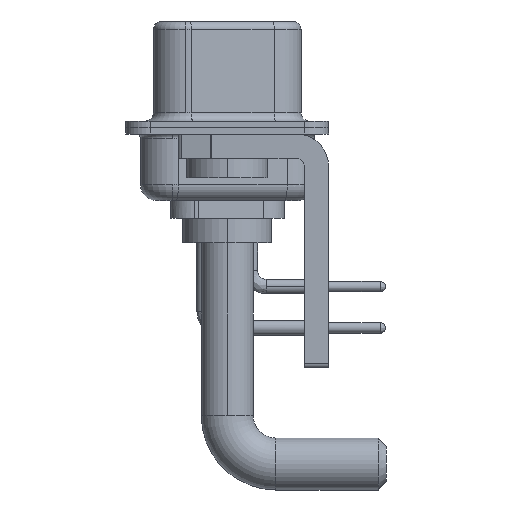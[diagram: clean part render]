
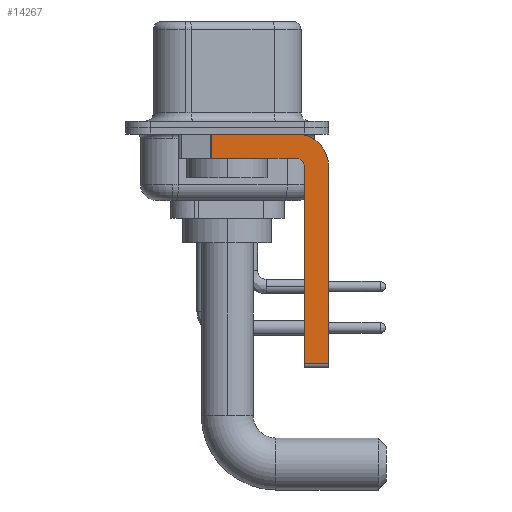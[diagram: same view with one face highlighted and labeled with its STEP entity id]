
A CAD part, left-side view. The second image highlights one B-rep face of the part: STEP entity #14267.
In plain terms, the highlighted planar face has unit normal (-1, 0, 0).
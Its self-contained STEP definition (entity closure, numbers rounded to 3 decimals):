
#264 = CARTESIAN_POINT ( 'NONE',  ( -2.9, -4.25, -1.9 ) ) ;
#725 = ORIENTED_EDGE ( 'NONE', *, *, #1832, .T. ) ;
#1237 = DIRECTION ( 'NONE',  ( 0., 0., -1. ) ) ;
#1832 = EDGE_CURVE ( 'NONE', #25204, #16708, #16396, .T. ) ;
#2020 = DIRECTION ( 'NONE',  ( -1., 0., 0. ) ) ;
#2712 = DIRECTION ( 'NONE',  ( 0., 1., 0. ) ) ;
#3116 = CARTESIAN_POINT ( 'NONE',  ( -2.9, -4.25, -0.4 ) ) ;
#3680 = EDGE_CURVE ( 'NONE', #15665, #16388, #22553, .T. ) ;
#3769 = VECTOR ( 'NONE', #4786, 1000. ) ;
#3960 = CARTESIAN_POINT ( 'NONE',  ( -2.9, -4.25, -2.4 ) ) ;
#3987 = VECTOR ( 'NONE', #17427, 1000. ) ;
#4106 = CARTESIAN_POINT ( 'NONE',  ( -2.9, -4.75, -2.4 ) ) ;
#4339 = DIRECTION ( 'NONE',  ( 0., 0., 1. ) ) ;
#4600 = AXIS2_PLACEMENT_3D ( 'NONE', #3960, #2020, #4339 ) ;
#4715 = AXIS2_PLACEMENT_3D ( 'NONE', #13512, #13131, #21506 ) ;
#4773 = LINE ( 'NONE', #264, #22095 ) ;
#4786 = DIRECTION ( 'NONE',  ( 0., -1., 0. ) ) ;
#5771 = CIRCLE ( 'NONE', #8228, 2. ) ;
#6760 = DIRECTION ( 'NONE',  ( 0., -1., 0. ) ) ;
#7414 = CARTESIAN_POINT ( 'NONE',  ( -2.9, -6.25, -2.4 ) ) ;
#8228 = AXIS2_PLACEMENT_3D ( 'NONE', #20189, #18760, #12455 ) ;
#8317 = CARTESIAN_POINT ( 'NONE',  ( -2.9, -6.25, -14.55 ) ) ;
#9466 = LINE ( 'NONE', #17308, #3987 ) ;
#10185 = LINE ( 'NONE', #18180, #3769 ) ;
#10259 = ORIENTED_EDGE ( 'NONE', *, *, #3680, .T. ) ;
#10865 = CARTESIAN_POINT ( 'NONE',  ( -2.9, -4.25, -1.9 ) ) ;
#11382 = LINE ( 'NONE', #7414, #23860 ) ;
#11461 = PLANE ( 'NONE',  #4715 ) ;
#12455 = DIRECTION ( 'NONE',  ( 0., 0., -1. ) ) ;
#12821 = VERTEX_POINT ( 'NONE', #3116 ) ;
#13131 = DIRECTION ( 'NONE',  ( 1., 0., 0. ) ) ;
#13512 = CARTESIAN_POINT ( 'NONE',  ( -2.9, -4.25, -2.4 ) ) ;
#13577 = VERTEX_POINT ( 'NONE', #4106 ) ;
#13723 = EDGE_LOOP ( 'NONE', ( #19848, #10259, #16728, #17466, #16295, #725, #15737, #25098 ) ) ;
#14267 = ADVANCED_FACE ( 'NONE', ( #17257 ), #11461, .F. ) ;
#14851 = CARTESIAN_POINT ( 'NONE',  ( -2.9, 0.978, -0.4 ) ) ;
#15204 = CARTESIAN_POINT ( 'NONE',  ( -2.9, 0.978, -1.9 ) ) ;
#15551 = VECTOR ( 'NONE', #6760, 1000. ) ;
#15665 = VERTEX_POINT ( 'NONE', #14851 ) ;
#15737 = ORIENTED_EDGE ( 'NONE', *, *, #23624, .F. ) ;
#16140 = CARTESIAN_POINT ( 'NONE',  ( -2.9, -4.25, -14.55 ) ) ;
#16295 = ORIENTED_EDGE ( 'NONE', *, *, #18803, .F. ) ;
#16300 = CARTESIAN_POINT ( 'NONE',  ( -2.9, 0.978, -1.9 ) ) ;
#16386 = CARTESIAN_POINT ( 'NONE',  ( -2.9, -4.75, -14.55 ) ) ;
#16388 = VERTEX_POINT ( 'NONE', #16300 ) ;
#16396 = LINE ( 'NONE', #16140, #15551 ) ;
#16708 = VERTEX_POINT ( 'NONE', #8317 ) ;
#16728 = ORIENTED_EDGE ( 'NONE', *, *, #19268, .F. ) ;
#16930 = VERTEX_POINT ( 'NONE', #10865 ) ;
#17257 = FACE_OUTER_BOUND ( 'NONE', #13723, .T. ) ;
#17308 = CARTESIAN_POINT ( 'NONE',  ( -2.9, -4.75, -14.8 ) ) ;
#17427 = DIRECTION ( 'NONE',  ( 0., 0., 1. ) ) ;
#17466 = ORIENTED_EDGE ( 'NONE', *, *, #24702, .F. ) ;
#18067 = VERTEX_POINT ( 'NONE', #24895 ) ;
#18180 = CARTESIAN_POINT ( 'NONE',  ( -2.9, 3., -0.4 ) ) ;
#18760 = DIRECTION ( 'NONE',  ( 1., 0., 0. ) ) ;
#18803 = EDGE_CURVE ( 'NONE', #25204, #13577, #9466, .T. ) ;
#18820 = DIRECTION ( 'NONE',  ( 0., 0., -1. ) ) ;
#19268 = EDGE_CURVE ( 'NONE', #16930, #16388, #4773, .T. ) ;
#19848 = ORIENTED_EDGE ( 'NONE', *, *, #24388, .F. ) ;
#20189 = CARTESIAN_POINT ( 'NONE',  ( -2.9, -4.25, -2.4 ) ) ;
#21506 = DIRECTION ( 'NONE',  ( 0., 0., -1. ) ) ;
#22014 = VECTOR ( 'NONE', #18820, 1000. ) ;
#22095 = VECTOR ( 'NONE', #2712, 1000. ) ;
#22553 = LINE ( 'NONE', #15204, #22014 ) ;
#23046 = EDGE_CURVE ( 'NONE', #12821, #18067, #5771, .T. ) ;
#23624 = EDGE_CURVE ( 'NONE', #18067, #16708, #11382, .T. ) ;
#23860 = VECTOR ( 'NONE', #1237, 1000. ) ;
#23900 = CIRCLE ( 'NONE', #4600, 0.5 ) ;
#24388 = EDGE_CURVE ( 'NONE', #15665, #12821, #10185, .T. ) ;
#24702 = EDGE_CURVE ( 'NONE', #13577, #16930, #23900, .T. ) ;
#24895 = CARTESIAN_POINT ( 'NONE',  ( -2.9, -6.25, -2.4 ) ) ;
#25098 = ORIENTED_EDGE ( 'NONE', *, *, #23046, .F. ) ;
#25204 = VERTEX_POINT ( 'NONE', #16386 ) ;
